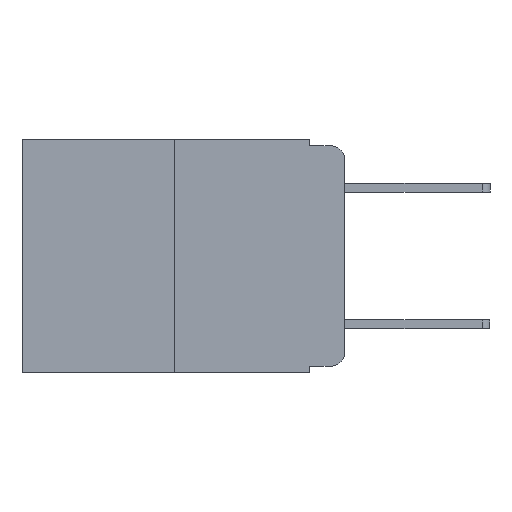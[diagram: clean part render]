
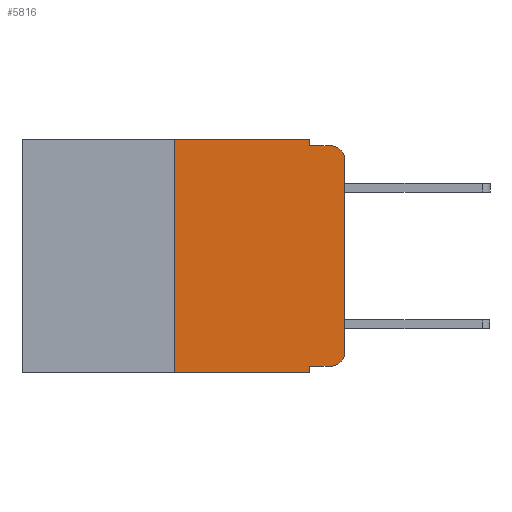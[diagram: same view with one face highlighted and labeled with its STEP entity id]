
A CAD part, left-side view. The second image highlights one B-rep face of the part: STEP entity #5816.
In plain terms, the highlighted planar face has unit normal (-1, 0, 0).
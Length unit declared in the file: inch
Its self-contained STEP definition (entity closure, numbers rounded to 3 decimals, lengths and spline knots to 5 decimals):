
#48 = ORIENTED_EDGE ( 'NONE', *, *, #8655, .T. ) ;
#105 = ORIENTED_EDGE ( 'NONE', *, *, #10401, .F. ) ;
#225 = ORIENTED_EDGE ( 'NONE', *, *, #604, .F. ) ;
#349 = EDGE_LOOP ( 'NONE', ( #2811, #4366, #4789, #5094, #105, #1503, #48, #225, #489, #533 ) ) ;
#428 = AXIS2_PLACEMENT_3D ( 'NONE', #4506, #10351, #5457 ) ;
#437 = DIRECTION ( 'NONE',  ( 0., 0., -1. ) ) ;
#489 = ORIENTED_EDGE ( 'NONE', *, *, #9653, .T. ) ;
#533 = ORIENTED_EDGE ( 'NONE', *, *, #4198, .T. ) ;
#572 = FACE_OUTER_BOUND ( 'NONE', #349, .T. ) ;
#604 = EDGE_CURVE ( 'NONE', #11176, #8489, #8277, .T. ) ;
#1023 = DIRECTION ( 'NONE',  ( 0., 0., -1. ) ) ;
#1503 = ORIENTED_EDGE ( 'NONE', *, *, #7520, .F. ) ;
#1534 = CARTESIAN_POINT ( 'NONE',  ( 0., 0.02, -0.01 ) ) ;
#1606 = CARTESIAN_POINT ( 'NONE',  ( 0., 0.051, -0.343 ) ) ;
#1970 = CARTESIAN_POINT ( 'NONE',  ( 0., 0.25, 0. ) ) ;
#2004 = VERTEX_POINT ( 'NONE', #8308 ) ;
#2360 = LINE ( 'NONE', #10486, #9229 ) ;
#2574 = CARTESIAN_POINT ( 'NONE',  ( 0., 0.051, -0.01 ) ) ;
#2811 = ORIENTED_EDGE ( 'NONE', *, *, #9379, .T. ) ;
#3218 = CARTESIAN_POINT ( 'NONE',  ( 0., 0.051, -0.333 ) ) ;
#3238 = CIRCLE ( 'NONE', #10347, 0.02 ) ;
#3370 = CARTESIAN_POINT ( 'NONE',  ( 0., 0.25, -0.343 ) ) ;
#3550 = CARTESIAN_POINT ( 'NONE',  ( 0., 0.051, -0.333 ) ) ;
#3682 = VERTEX_POINT ( 'NONE', #7854 ) ;
#3913 = VECTOR ( 'NONE', #8058, 39.37008 ) ;
#4198 = EDGE_CURVE ( 'NONE', #2004, #7352, #10124, .T. ) ;
#4366 = ORIENTED_EDGE ( 'NONE', *, *, #7293, .T. ) ;
#4506 = CARTESIAN_POINT ( 'NONE',  ( 0., 0.02, -0.313 ) ) ;
#4577 = EDGE_CURVE ( 'NONE', #3682, #10186, #9069, .T. ) ;
#4761 = DIRECTION ( 'NONE',  ( 0., -1., 0. ) ) ;
#4789 = ORIENTED_EDGE ( 'NONE', *, *, #9887, .F. ) ;
#4884 = VECTOR ( 'NONE', #6509, 39.37008 ) ;
#5094 = ORIENTED_EDGE ( 'NONE', *, *, #4577, .F. ) ;
#5350 = CARTESIAN_POINT ( 'NONE',  ( 0., 0.473, 0. ) ) ;
#5400 = LINE ( 'NONE', #6241, #9575 ) ;
#5457 = DIRECTION ( 'NONE',  ( 0., 0., -1. ) ) ;
#5704 = CARTESIAN_POINT ( 'NONE',  ( 0., 0.473, -0.343 ) ) ;
#5816 = ADVANCED_FACE ( 'NONE', ( #572 ), #10241, .F. ) ;
#5884 = CARTESIAN_POINT ( 'NONE',  ( 0., 0.25, 0. ) ) ;
#6012 = VECTOR ( 'NONE', #11382, 39.37008 ) ;
#6241 = CARTESIAN_POINT ( 'NONE',  ( 0., 0., 0. ) ) ;
#6277 = VERTEX_POINT ( 'NONE', #3370 ) ;
#6323 = DIRECTION ( 'NONE',  ( 0., 0., -1. ) ) ;
#6509 = DIRECTION ( 'NONE',  ( 0., -1., 0. ) ) ;
#6610 = DIRECTION ( 'NONE',  ( -1., 0., 0. ) ) ;
#6853 = DIRECTION ( 'NONE',  ( 0., 0., 1. ) ) ;
#6977 = VECTOR ( 'NONE', #1023, 39.37008 ) ;
#7106 = CARTESIAN_POINT ( 'NONE',  ( 0., 0.051, 0. ) ) ;
#7293 = EDGE_CURVE ( 'NONE', #7528, #9797, #3238, .T. ) ;
#7352 = VERTEX_POINT ( 'NONE', #7466 ) ;
#7370 = CARTESIAN_POINT ( 'NONE',  ( 0., 0.473, 0. ) ) ;
#7466 = CARTESIAN_POINT ( 'NONE',  ( 0., 0., -0.313 ) ) ;
#7520 = EDGE_CURVE ( 'NONE', #6277, #7531, #9941, .T. ) ;
#7528 = VERTEX_POINT ( 'NONE', #7670 ) ;
#7531 = VERTEX_POINT ( 'NONE', #1970 ) ;
#7649 = LINE ( 'NONE', #5704, #11214 ) ;
#7670 = CARTESIAN_POINT ( 'NONE',  ( 0., 0., -0.03 ) ) ;
#7808 = CARTESIAN_POINT ( 'NONE',  ( 0., 0.051, 0. ) ) ;
#7854 = CARTESIAN_POINT ( 'NONE',  ( 0., 0.051, 0. ) ) ;
#7889 = VECTOR ( 'NONE', #6853, 39.37008 ) ;
#8058 = DIRECTION ( 'NONE',  ( 0., -1., 0. ) ) ;
#8277 = LINE ( 'NONE', #7106, #6012 ) ;
#8308 = CARTESIAN_POINT ( 'NONE',  ( 0., 0.02, -0.333 ) ) ;
#8489 = VERTEX_POINT ( 'NONE', #1606 ) ;
#8655 = EDGE_CURVE ( 'NONE', #6277, #8489, #7649, .T. ) ;
#9069 = LINE ( 'NONE', #7808, #6977 ) ;
#9229 = VECTOR ( 'NONE', #11238, 39.37008 ) ;
#9379 = EDGE_CURVE ( 'NONE', #7352, #7528, #5400, .T. ) ;
#9575 = VECTOR ( 'NONE', #11710, 39.37008 ) ;
#9653 = EDGE_CURVE ( 'NONE', #11176, #2004, #10645, .T. ) ;
#9797 = VERTEX_POINT ( 'NONE', #1534 ) ;
#9887 = EDGE_CURVE ( 'NONE', #10186, #9797, #2360, .T. ) ;
#9941 = LINE ( 'NONE', #5884, #7889 ) ;
#10124 = CIRCLE ( 'NONE', #428, 0.02 ) ;
#10186 = VERTEX_POINT ( 'NONE', #2574 ) ;
#10202 = AXIS2_PLACEMENT_3D ( 'NONE', #5350, #11033, #6323 ) ;
#10241 = PLANE ( 'NONE',  #10202 ) ;
#10347 = AXIS2_PLACEMENT_3D ( 'NONE', #11263, #6610, #437 ) ;
#10351 = DIRECTION ( 'NONE',  ( -1., 0., 0. ) ) ;
#10401 = EDGE_CURVE ( 'NONE', #7531, #3682, #11405, .T. ) ;
#10486 = CARTESIAN_POINT ( 'NONE',  ( 0., 0.051, -0.01 ) ) ;
#10645 = LINE ( 'NONE', #3550, #3913 ) ;
#11033 = DIRECTION ( 'NONE',  ( 1., 0., 0. ) ) ;
#11176 = VERTEX_POINT ( 'NONE', #3218 ) ;
#11214 = VECTOR ( 'NONE', #4761, 39.37008 ) ;
#11238 = DIRECTION ( 'NONE',  ( 0., -1., 0. ) ) ;
#11263 = CARTESIAN_POINT ( 'NONE',  ( 0., 0.02, -0.03 ) ) ;
#11382 = DIRECTION ( 'NONE',  ( 0., 0., -1. ) ) ;
#11405 = LINE ( 'NONE', #7370, #4884 ) ;
#11710 = DIRECTION ( 'NONE',  ( 0., 0., 1. ) ) ;
